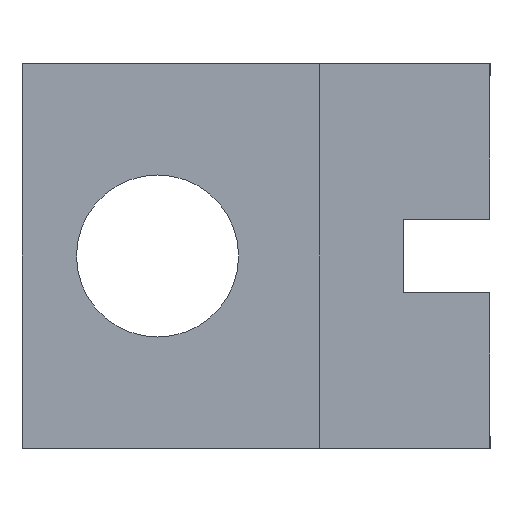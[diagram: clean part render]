
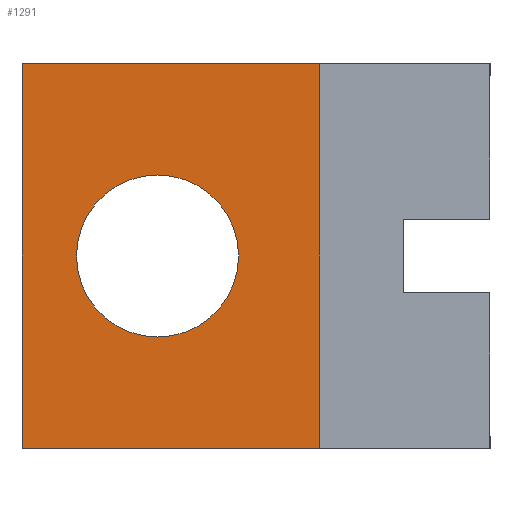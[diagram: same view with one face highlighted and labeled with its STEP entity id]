
A CAD part, front view. The second image highlights one B-rep face of the part: STEP entity #1291.
In plain terms, the highlighted planar face has unit normal (0, -1, 0).
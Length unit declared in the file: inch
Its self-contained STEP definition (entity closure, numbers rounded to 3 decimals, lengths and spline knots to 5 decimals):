
#5 = DIRECTION ( 'NONE',  ( 0., 0., -1. ) ) ;
#23 = DIRECTION ( 'NONE',  ( 0., 1., 0. ) ) ;
#28 = AXIS2_PLACEMENT_3D ( 'NONE', #575, #188, #983 ) ;
#49 = DIRECTION ( 'NONE',  ( 1., 0., 0. ) ) ;
#56 = DIRECTION ( 'NONE',  ( 1., 0., 0. ) ) ;
#95 = VECTOR ( 'NONE', #926, 39.37008 ) ;
#98 = DIRECTION ( 'NONE',  ( 0., -1., 0. ) ) ;
#111 = AXIS2_PLACEMENT_3D ( 'NONE', #527, #23, #1315 ) ;
#146 = EDGE_CURVE ( 'NONE', #1177, #280, #633, .T. ) ;
#171 = CARTESIAN_POINT ( 'NONE',  ( 0.2865, 0., 0.37 ) ) ;
#177 = CARTESIAN_POINT ( 'NONE',  ( 0., 0., 0.37 ) ) ;
#188 = DIRECTION ( 'NONE',  ( 0., -1., 0. ) ) ;
#208 = ORIENTED_EDGE ( 'NONE', *, *, #400, .F. ) ;
#216 = CARTESIAN_POINT ( 'NONE',  ( 0.2865, 0., 0.37 ) ) ;
#241 = EDGE_CURVE ( 'NONE', #799, #572, #1088, .T. ) ;
#280 = VERTEX_POINT ( 'NONE', #568 ) ;
#317 = EDGE_CURVE ( 'NONE', #1079, #1277, #776, .T. ) ;
#353 = CARTESIAN_POINT ( 'NONE',  ( 0., 0., 0. ) ) ;
#388 = EDGE_CURVE ( 'NONE', #1277, #1079, #1013, .T. ) ;
#400 = EDGE_CURVE ( 'NONE', #572, #280, #913, .T. ) ;
#405 = CARTESIAN_POINT ( 'NONE',  ( 0., 0., 0.37 ) ) ;
#449 = EDGE_LOOP ( 'NONE', ( #1233, #706 ) ) ;
#506 = VECTOR ( 'NONE', #49, 39.37008 ) ;
#527 = CARTESIAN_POINT ( 'NONE',  ( 0., 0., 0.37 ) ) ;
#568 = CARTESIAN_POINT ( 'NONE',  ( 0.2865, 0., 0. ) ) ;
#572 = VERTEX_POINT ( 'NONE', #171 ) ;
#575 = CARTESIAN_POINT ( 'NONE',  ( 0.1305, 0., 0.185 ) ) ;
#601 = ORIENTED_EDGE ( 'NONE', *, *, #241, .F. ) ;
#609 = CARTESIAN_POINT ( 'NONE',  ( 0.1305, 0., 0.185 ) ) ;
#614 = PLANE ( 'NONE',  #111 ) ;
#633 = LINE ( 'NONE', #353, #506 ) ;
#666 = CARTESIAN_POINT ( 'NONE',  ( 0., 0., 0.37 ) ) ;
#706 = ORIENTED_EDGE ( 'NONE', *, *, #317, .F. ) ;
#765 = LINE ( 'NONE', #177, #95 ) ;
#776 = CIRCLE ( 'NONE', #28, 0.078 ) ;
#777 = EDGE_LOOP ( 'NONE', ( #1064, #208, #601, #1029 ) ) ;
#799 = VERTEX_POINT ( 'NONE', #405 ) ;
#905 = CARTESIAN_POINT ( 'NONE',  ( 0., 0., 0. ) ) ;
#913 = LINE ( 'NONE', #216, #1307 ) ;
#926 = DIRECTION ( 'NONE',  ( 0., 0., -1. ) ) ;
#931 = VECTOR ( 'NONE', #56, 39.37008 ) ;
#940 = FACE_BOUND ( 'NONE', #449, .T. ) ;
#943 = FACE_OUTER_BOUND ( 'NONE', #777, .T. ) ;
#982 = EDGE_CURVE ( 'NONE', #799, #1177, #765, .T. ) ;
#983 = DIRECTION ( 'NONE',  ( -1., 0., 0. ) ) ;
#1013 = CIRCLE ( 'NONE', #1205, 0.078 ) ;
#1015 = CARTESIAN_POINT ( 'NONE',  ( 0.1305, 0., 0.263 ) ) ;
#1017 = DIRECTION ( 'NONE',  ( -1., 0., 0. ) ) ;
#1029 = ORIENTED_EDGE ( 'NONE', *, *, #982, .T. ) ;
#1064 = ORIENTED_EDGE ( 'NONE', *, *, #146, .T. ) ;
#1069 = CARTESIAN_POINT ( 'NONE',  ( 0.1305, 0., 0.107 ) ) ;
#1079 = VERTEX_POINT ( 'NONE', #1069 ) ;
#1088 = LINE ( 'NONE', #666, #931 ) ;
#1177 = VERTEX_POINT ( 'NONE', #905 ) ;
#1205 = AXIS2_PLACEMENT_3D ( 'NONE', #609, #98, #1017 ) ;
#1233 = ORIENTED_EDGE ( 'NONE', *, *, #388, .F. ) ;
#1277 = VERTEX_POINT ( 'NONE', #1015 ) ;
#1291 = ADVANCED_FACE ( 'NONE', ( #943, #940 ), #614, .F. ) ;
#1307 = VECTOR ( 'NONE', #5, 39.37008 ) ;
#1315 = DIRECTION ( 'NONE',  ( -1., 0., 0. ) ) ;
